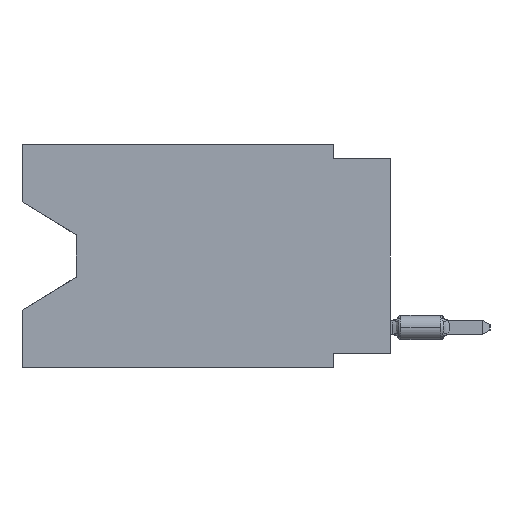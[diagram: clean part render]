
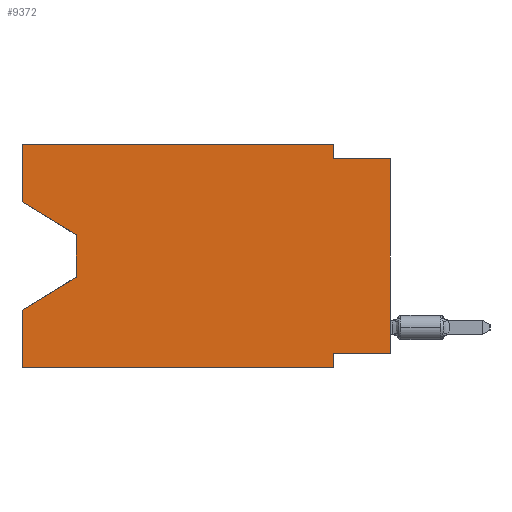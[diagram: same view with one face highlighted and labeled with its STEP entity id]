
A CAD part, left-side view. The second image highlights one B-rep face of the part: STEP entity #9372.
In plain terms, the highlighted planar face has unit normal (-1, 0, 0).
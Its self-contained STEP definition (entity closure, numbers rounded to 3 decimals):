
#493 = LINE ( 'NONE', #16354, #33188 ) ;
#592 = LINE ( 'NONE', #23271, #28815 ) ;
#2166 = AXIS2_PLACEMENT_3D ( 'NONE', #18557, #23555, #34397 ) ;
#2286 = VERTEX_POINT ( 'NONE', #12982 ) ;
#3189 = ORIENTED_EDGE ( 'NONE', *, *, #28766, .T. ) ;
#3435 = ORIENTED_EDGE ( 'NONE', *, *, #47302, .F. ) ;
#5879 = CARTESIAN_POINT ( 'NONE',  ( 0., 16.383, 0. ) ) ;
#6133 = VECTOR ( 'NONE', #7002, 1000. ) ;
#7002 = DIRECTION ( 'NONE',  ( 0., -1., 0. ) ) ;
#7073 = VERTEX_POINT ( 'NONE', #30277 ) ;
#8021 = VERTEX_POINT ( 'NONE', #41217 ) ;
#9248 = ORIENTED_EDGE ( 'NONE', *, *, #43748, .F. ) ;
#9372 = ADVANCED_FACE ( 'NONE', ( #38420 ), #27314, .F. ) ;
#9630 = ORIENTED_EDGE ( 'NONE', *, *, #31143, .F. ) ;
#10154 = CARTESIAN_POINT ( 'NONE',  ( 0., 2.54, 0. ) ) ;
#11314 = VECTOR ( 'NONE', #43705, 1000. ) ;
#11386 = VECTOR ( 'NONE', #42956, 1000. ) ;
#11766 = LINE ( 'NONE', #34447, #17204 ) ;
#12508 = ORIENTED_EDGE ( 'NONE', *, *, #24842, .F. ) ;
#12622 = VERTEX_POINT ( 'NONE', #48765 ) ;
#12643 = VERTEX_POINT ( 'NONE', #14530 ) ;
#12685 = EDGE_CURVE ( 'NONE', #12643, #33550, #20023, .T. ) ;
#12846 = CARTESIAN_POINT ( 'NONE',  ( 0., 2.54, -9.271 ) ) ;
#12982 = CARTESIAN_POINT ( 'NONE',  ( 0., 0., -0.635 ) ) ;
#13282 = DIRECTION ( 'NONE',  ( 0., 1., 0. ) ) ;
#13596 = VERTEX_POINT ( 'NONE', #21097 ) ;
#13707 = VECTOR ( 'NONE', #46001, 1000. ) ;
#13733 = VECTOR ( 'NONE', #47861, 1000. ) ;
#14530 = CARTESIAN_POINT ( 'NONE',  ( 0., 13.97, -5.893 ) ) ;
#15302 = EDGE_CURVE ( 'NONE', #12622, #2286, #493, .T. ) ;
#16354 = CARTESIAN_POINT ( 'NONE',  ( 0., 0., 0. ) ) ;
#17038 = EDGE_CURVE ( 'NONE', #8021, #12643, #33148, .T. ) ;
#17159 = LINE ( 'NONE', #32491, #13733 ) ;
#17204 = VECTOR ( 'NONE', #49556, 1000. ) ;
#18557 = CARTESIAN_POINT ( 'NONE',  ( 0., 16.383, 0. ) ) ;
#18951 = EDGE_CURVE ( 'NONE', #26880, #7073, #40323, .T. ) ;
#19909 = ORIENTED_EDGE ( 'NONE', *, *, #17038, .T. ) ;
#20023 = LINE ( 'NONE', #27784, #13707 ) ;
#20199 = VERTEX_POINT ( 'NONE', #39757 ) ;
#20570 = ORIENTED_EDGE ( 'NONE', *, *, #12685, .T. ) ;
#21097 = CARTESIAN_POINT ( 'NONE',  ( 0., 16.383, -9.906 ) ) ;
#22320 = VERTEX_POINT ( 'NONE', #10154 ) ;
#23271 = CARTESIAN_POINT ( 'NONE',  ( 0., 16.383, 0. ) ) ;
#23345 = CARTESIAN_POINT ( 'NONE',  ( 0., 16.383, 0. ) ) ;
#23555 = DIRECTION ( 'NONE',  ( 1., 0., 0. ) ) ;
#24842 = EDGE_CURVE ( 'NONE', #20199, #28848, #592, .T. ) ;
#25249 = ORIENTED_EDGE ( 'NONE', *, *, #18951, .F. ) ;
#25331 = CARTESIAN_POINT ( 'NONE',  ( 0., 13.97, -4.013 ) ) ;
#25436 = CARTESIAN_POINT ( 'NONE',  ( 0., 2.54, -9.906 ) ) ;
#26615 = VECTOR ( 'NONE', #13282, 1000. ) ;
#26880 = VERTEX_POINT ( 'NONE', #12846 ) ;
#27314 = PLANE ( 'NONE',  #2166 ) ;
#27519 = DIRECTION ( 'NONE',  ( 0., 0., 1. ) ) ;
#27784 = CARTESIAN_POINT ( 'NONE',  ( 0., 13.97, -5.893 ) ) ;
#28380 = CARTESIAN_POINT ( 'NONE',  ( 0., 0., -9.271 ) ) ;
#28577 = ORIENTED_EDGE ( 'NONE', *, *, #46343, .F. ) ;
#28766 = EDGE_CURVE ( 'NONE', #20199, #8021, #17159, .T. ) ;
#28815 = VECTOR ( 'NONE', #27519, 1000. ) ;
#28848 = VERTEX_POINT ( 'NONE', #23345 ) ;
#29629 = CARTESIAN_POINT ( 'NONE',  ( 0., 16.383, -9.906 ) ) ;
#30215 = ORIENTED_EDGE ( 'NONE', *, *, #46985, .F. ) ;
#30277 = CARTESIAN_POINT ( 'NONE',  ( 0., 2.54, -9.906 ) ) ;
#31143 = EDGE_CURVE ( 'NONE', #38164, #2286, #11766, .T. ) ;
#32316 = ORIENTED_EDGE ( 'NONE', *, *, #15302, .T. ) ;
#32491 = CARTESIAN_POINT ( 'NONE',  ( 0., 16.383, -2.546 ) ) ;
#32501 = EDGE_LOOP ( 'NONE', ( #3189, #19909, #20570, #28577, #37725, #25249, #30215, #32316, #9630, #3435, #9248, #12508 ) ) ;
#32835 = LINE ( 'NONE', #5879, #11314 ) ;
#33148 = LINE ( 'NONE', #25331, #48629 ) ;
#33188 = VECTOR ( 'NONE', #39247, 1000. ) ;
#33550 = VERTEX_POINT ( 'NONE', #48584 ) ;
#34397 = DIRECTION ( 'NONE',  ( 0., 0., -1. ) ) ;
#34447 = CARTESIAN_POINT ( 'NONE',  ( 0., 0., -0.635 ) ) ;
#36325 = VECTOR ( 'NONE', #45017, 1000. ) ;
#36426 = DIRECTION ( 'NONE',  ( 0., 0., -1. ) ) ;
#36446 = LINE ( 'NONE', #28380, #26615 ) ;
#37725 = ORIENTED_EDGE ( 'NONE', *, *, #47254, .T. ) ;
#38164 = VERTEX_POINT ( 'NONE', #48644 ) ;
#38420 = FACE_OUTER_BOUND ( 'NONE', #32501, .T. ) ;
#39247 = DIRECTION ( 'NONE',  ( 0., 0., 1. ) ) ;
#39757 = CARTESIAN_POINT ( 'NONE',  ( 0., 16.383, -2.546 ) ) ;
#40323 = LINE ( 'NONE', #25436, #43128 ) ;
#40816 = DIRECTION ( 'NONE',  ( 0., 0., -1. ) ) ;
#41217 = CARTESIAN_POINT ( 'NONE',  ( 0., 13.97, -4.013 ) ) ;
#42956 = DIRECTION ( 'NONE',  ( 0., 0., -1. ) ) ;
#43128 = VECTOR ( 'NONE', #40816, 1000. ) ;
#43705 = DIRECTION ( 'NONE',  ( 0., 0., 1. ) ) ;
#43748 = EDGE_CURVE ( 'NONE', #28848, #22320, #48842, .T. ) ;
#45017 = DIRECTION ( 'NONE',  ( 0., -1., 0. ) ) ;
#45339 = CARTESIAN_POINT ( 'NONE',  ( 0., 16.383, 0. ) ) ;
#45517 = LINE ( 'NONE', #29629, #36325 ) ;
#46001 = DIRECTION ( 'NONE',  ( 0., 0.855, -0.519 ) ) ;
#46252 = CARTESIAN_POINT ( 'NONE',  ( 0., 2.54, 0. ) ) ;
#46343 = EDGE_CURVE ( 'NONE', #13596, #33550, #32835, .T. ) ;
#46985 = EDGE_CURVE ( 'NONE', #12622, #26880, #36446, .T. ) ;
#47219 = LINE ( 'NONE', #46252, #11386 ) ;
#47254 = EDGE_CURVE ( 'NONE', #13596, #7073, #45517, .T. ) ;
#47302 = EDGE_CURVE ( 'NONE', #22320, #38164, #47219, .T. ) ;
#47861 = DIRECTION ( 'NONE',  ( 0., -0.855, -0.519 ) ) ;
#48584 = CARTESIAN_POINT ( 'NONE',  ( 0., 16.383, -7.36 ) ) ;
#48629 = VECTOR ( 'NONE', #36426, 1000. ) ;
#48644 = CARTESIAN_POINT ( 'NONE',  ( 0., 2.54, -0.635 ) ) ;
#48765 = CARTESIAN_POINT ( 'NONE',  ( 0., 0., -9.271 ) ) ;
#48842 = LINE ( 'NONE', #45339, #6133 ) ;
#49556 = DIRECTION ( 'NONE',  ( 0., -1., 0. ) ) ;
